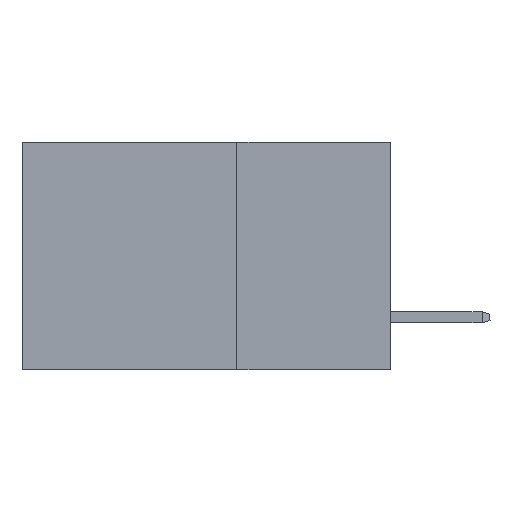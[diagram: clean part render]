
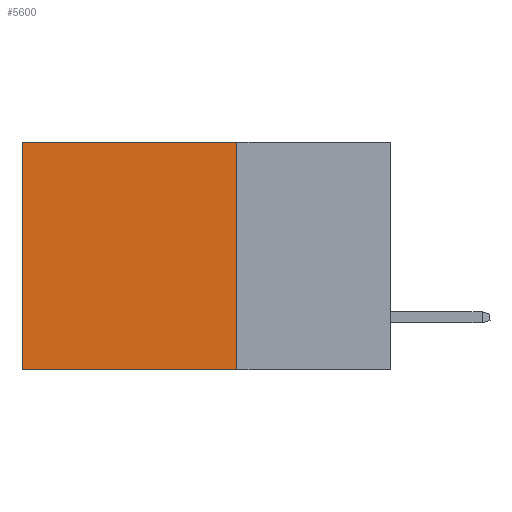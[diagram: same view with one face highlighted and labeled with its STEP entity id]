
A CAD part, left-side view. The second image highlights one B-rep face of the part: STEP entity #5600.
In plain terms, the highlighted planar face has unit normal (-1, 0, 0).
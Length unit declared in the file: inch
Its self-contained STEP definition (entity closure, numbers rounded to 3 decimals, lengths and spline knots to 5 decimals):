
#3095 = CARTESIAN_POINT ( 'NONE',  ( 0.2875, 0.25, 0. ) ) ;
#4942 = VERTEX_POINT ( 'NONE', #8677 ) ;
#5339 = CARTESIAN_POINT ( 'NONE',  ( 0.2875, 0.25, 0. ) ) ;
#5600 = ADVANCED_FACE ( 'NONE', ( #6302 ), #17229, .F. ) ;
#5719 = CARTESIAN_POINT ( 'NONE',  ( 0.2875, 0.6, 0. ) ) ;
#6302 = FACE_OUTER_BOUND ( 'NONE', #36512, .T. ) ;
#7114 = VECTOR ( 'NONE', #13858, 39.37008 ) ;
#7190 = CARTESIAN_POINT ( 'NONE',  ( 0.2875, 0.6, 0. ) ) ;
#8677 = CARTESIAN_POINT ( 'NONE',  ( 0.2875, 0.25, -0.37 ) ) ;
#9260 = VECTOR ( 'NONE', #22097, 39.37008 ) ;
#10067 = VECTOR ( 'NONE', #14464, 39.37008 ) ;
#10782 = VECTOR ( 'NONE', #12870, 39.37008 ) ;
#11717 = DIRECTION ( 'NONE',  ( 1., 0., 0. ) ) ;
#12232 = CARTESIAN_POINT ( 'NONE',  ( 0.2875, 0.6, -0.37 ) ) ;
#12870 = DIRECTION ( 'NONE',  ( 0., 0., -1. ) ) ;
#13289 = ORIENTED_EDGE ( 'NONE', *, *, #26548, .F. ) ;
#13858 = DIRECTION ( 'NONE',  ( 0., 1., 0. ) ) ;
#14464 = DIRECTION ( 'NONE',  ( 0., 0., -1. ) ) ;
#14611 = LINE ( 'NONE', #5339, #7114 ) ;
#15609 = VERTEX_POINT ( 'NONE', #26101 ) ;
#17229 = PLANE ( 'NONE',  #26288 ) ;
#18260 = LINE ( 'NONE', #7190, #10782 ) ;
#18316 = ORIENTED_EDGE ( 'NONE', *, *, #25662, .F. ) ;
#22097 = DIRECTION ( 'NONE',  ( 0., 1., 0. ) ) ;
#23120 = EDGE_CURVE ( 'NONE', #35422, #34129, #18260, .T. ) ;
#23183 = ORIENTED_EDGE ( 'NONE', *, *, #24680, .T. ) ;
#24680 = EDGE_CURVE ( 'NONE', #15609, #35422, #14611, .T. ) ;
#25042 = LINE ( 'NONE', #33338, #9260 ) ;
#25662 = EDGE_CURVE ( 'NONE', #4942, #34129, #25042, .T. ) ;
#26101 = CARTESIAN_POINT ( 'NONE',  ( 0.2875, 0.25, 0. ) ) ;
#26288 = AXIS2_PLACEMENT_3D ( 'NONE', #28529, #11717, #31384 ) ;
#26548 = EDGE_CURVE ( 'NONE', #15609, #4942, #32533, .T. ) ;
#28529 = CARTESIAN_POINT ( 'NONE',  ( 0.2875, 0.25, 0. ) ) ;
#31384 = DIRECTION ( 'NONE',  ( 0., 0., -1. ) ) ;
#32533 = LINE ( 'NONE', #3095, #10067 ) ;
#33338 = CARTESIAN_POINT ( 'NONE',  ( 0.2875, 0.25, -0.37 ) ) ;
#34129 = VERTEX_POINT ( 'NONE', #12232 ) ;
#34825 = ORIENTED_EDGE ( 'NONE', *, *, #23120, .T. ) ;
#35422 = VERTEX_POINT ( 'NONE', #5719 ) ;
#36512 = EDGE_LOOP ( 'NONE', ( #34825, #18316, #13289, #23183 ) ) ;
